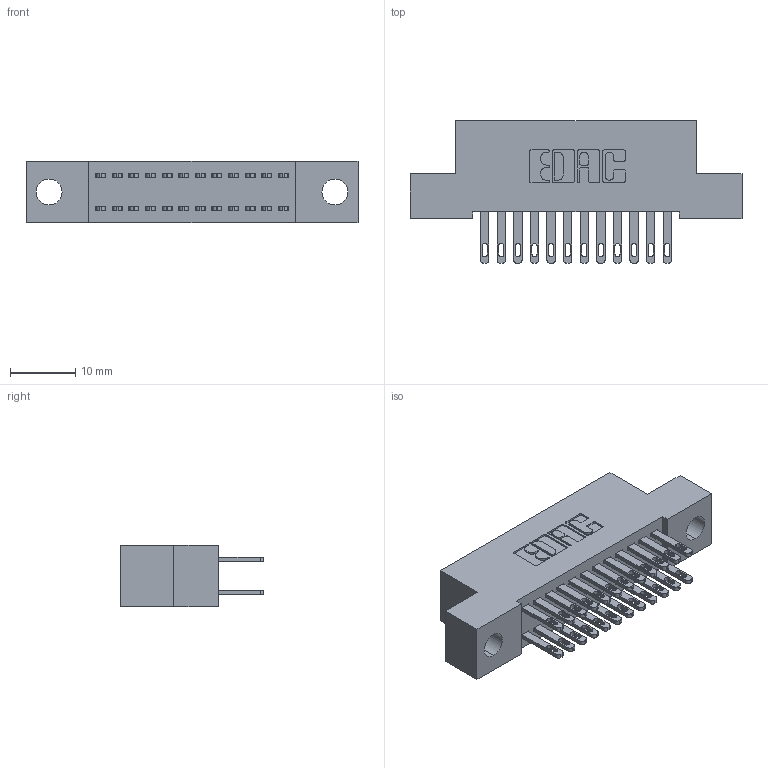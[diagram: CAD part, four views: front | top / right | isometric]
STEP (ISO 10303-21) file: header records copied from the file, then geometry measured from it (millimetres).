
FILE_DESCRIPTION (( 'STEP AP203' ), '1' );
FILE_NAME ('892-024-500-204.STEP', '2020-09-21T14:26:38', ( '' ), ( '' ), 'SwSTEP 2.0', 'SolidWorks 2020', '' );
FILE_SCHEMA (( 'CONFIG_CONTROL_DESIGN' ));
Length unit declared in the file: inch
Products named in the file (3): 892-024-500-204; 842 Part_.156 TH; 345-292-001_345-293-100
Assembly tree (25 placements, depth 2):
  892-024-500-204
    842 Part_.156 TH
    345-292-001_345-293-100  x24
Bounding box: 50.8 x 21.85 x 9.4 mm (x, y, z)
Volume: 4408.7 mm3; surface area: 6491 mm2
Topology: 25 solids, 25 shells, 1262 faces, 3827 edges, 2550 vertices
Faces by surface type: plane 786, cylinder 476
Entity records: 11401 total; most frequent: CARTESIAN_POINT 1922, ORIENTED_EDGE 1858, DIRECTION 1697, EDGE_CURVE 929, VECTOR 797, LINE 797, VERTEX_POINT 618, AXIS2_PLACEMENT_3D 450
